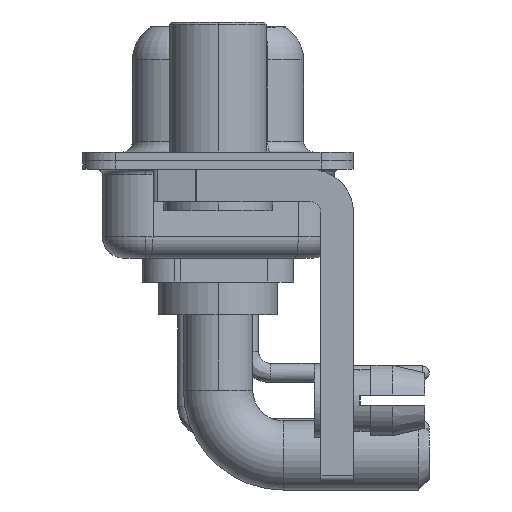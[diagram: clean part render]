
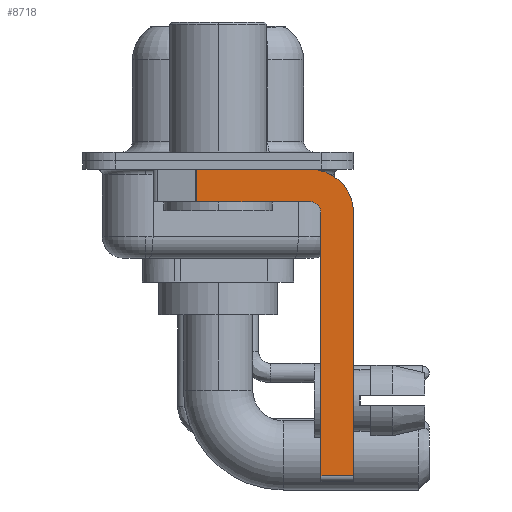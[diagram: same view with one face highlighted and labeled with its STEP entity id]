
A CAD part, left-side view. The second image highlights one B-rep face of the part: STEP entity #8718.
In plain terms, the highlighted planar face has unit normal (-1, 0, 0).
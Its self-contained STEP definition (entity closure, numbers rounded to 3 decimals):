
#2 = VECTOR ( 'NONE', #26113, 1000. ) ;
#580 = ORIENTED_EDGE ( 'NONE', *, *, #16286, .F. ) ;
#1079 = CIRCLE ( 'NONE', #10155, 2. ) ;
#2618 = DIRECTION ( 'NONE',  ( -1., 0., 0. ) ) ;
#2650 = CARTESIAN_POINT ( 'NONE',  ( -2.9, 0.978, -1.9 ) ) ;
#2651 = DIRECTION ( 'NONE',  ( 0., 0., 1. ) ) ;
#2759 = DIRECTION ( 'NONE',  ( 0., 0., -1. ) ) ;
#2904 = LINE ( 'NONE', #5308, #8463 ) ;
#2983 = ORIENTED_EDGE ( 'NONE', *, *, #18444, .F. ) ;
#3785 = DIRECTION ( 'NONE',  ( 1., 0., 0. ) ) ;
#4225 = DIRECTION ( 'NONE',  ( 0., -1., 0. ) ) ;
#4258 = VERTEX_POINT ( 'NONE', #25915 ) ;
#4605 = LINE ( 'NONE', #6196, #2 ) ;
#4687 = VERTEX_POINT ( 'NONE', #11005 ) ;
#4755 = DIRECTION ( 'NONE',  ( 0., 0., 1. ) ) ;
#4996 = CIRCLE ( 'NONE', #17217, 0.5 ) ;
#5308 = CARTESIAN_POINT ( 'NONE',  ( -2.9, 0.978, -1.9 ) ) ;
#5405 = EDGE_CURVE ( 'NONE', #19166, #7713, #22837, .T. ) ;
#5461 = EDGE_CURVE ( 'NONE', #7713, #22193, #1079, .T. ) ;
#5554 = DIRECTION ( 'NONE',  ( 0., -1., 0. ) ) ;
#6196 = CARTESIAN_POINT ( 'NONE',  ( -2.9, -6.25, -2.4 ) ) ;
#7471 = CARTESIAN_POINT ( 'NONE',  ( -2.9, -4.75, -14.8 ) ) ;
#7614 = DIRECTION ( 'NONE',  ( 0., 0., -1. ) ) ;
#7713 = VERTEX_POINT ( 'NONE', #16650 ) ;
#8463 = VECTOR ( 'NONE', #2759, 1000. ) ;
#8718 = ADVANCED_FACE ( 'NONE', ( #16398 ), #14412, .F. ) ;
#8815 = ORIENTED_EDGE ( 'NONE', *, *, #15920, .F. ) ;
#9011 = CARTESIAN_POINT ( 'NONE',  ( -2.9, -4.25, -2.4 ) ) ;
#10112 = ORIENTED_EDGE ( 'NONE', *, *, #24774, .F. ) ;
#10155 = AXIS2_PLACEMENT_3D ( 'NONE', #23113, #27479, #12633 ) ;
#10220 = CARTESIAN_POINT ( 'NONE',  ( -2.9, -6.25, -2.4 ) ) ;
#11005 = CARTESIAN_POINT ( 'NONE',  ( -2.9, -6.25, -14.55 ) ) ;
#11043 = LINE ( 'NONE', #26287, #24682 ) ;
#11050 = VECTOR ( 'NONE', #5554, 1000. ) ;
#11051 = CARTESIAN_POINT ( 'NONE',  ( -2.9, 0.978, -0.4 ) ) ;
#11721 = DIRECTION ( 'NONE',  ( 0., 1., 0. ) ) ;
#12083 = AXIS2_PLACEMENT_3D ( 'NONE', #25297, #3785, #7614 ) ;
#12367 = VERTEX_POINT ( 'NONE', #24842 ) ;
#12633 = DIRECTION ( 'NONE',  ( 0., 0., -1. ) ) ;
#13818 = VECTOR ( 'NONE', #11721, 1000. ) ;
#14412 = PLANE ( 'NONE',  #12083 ) ;
#15465 = ORIENTED_EDGE ( 'NONE', *, *, #5405, .F. ) ;
#15551 = ORIENTED_EDGE ( 'NONE', *, *, #25439, .T. ) ;
#15710 = CARTESIAN_POINT ( 'NONE',  ( -2.9, -4.25, -1.9 ) ) ;
#15920 = EDGE_CURVE ( 'NONE', #4258, #17769, #20084, .T. ) ;
#16286 = EDGE_CURVE ( 'NONE', #22193, #4687, #4605, .T. ) ;
#16398 = FACE_OUTER_BOUND ( 'NONE', #22887, .T. ) ;
#16650 = CARTESIAN_POINT ( 'NONE',  ( -2.9, -4.25, -0.4 ) ) ;
#17217 = AXIS2_PLACEMENT_3D ( 'NONE', #9011, #2618, #4755 ) ;
#17769 = VERTEX_POINT ( 'NONE', #25462 ) ;
#18152 = ORIENTED_EDGE ( 'NONE', *, *, #5461, .F. ) ;
#18444 = EDGE_CURVE ( 'NONE', #17769, #12367, #4996, .T. ) ;
#18498 = ORIENTED_EDGE ( 'NONE', *, *, #24621, .T. ) ;
#19166 = VERTEX_POINT ( 'NONE', #11051 ) ;
#20084 = LINE ( 'NONE', #7471, #23036 ) ;
#22193 = VERTEX_POINT ( 'NONE', #10220 ) ;
#22837 = LINE ( 'NONE', #24945, #11050 ) ;
#22887 = EDGE_LOOP ( 'NONE', ( #15465, #15551, #10112, #2983, #8815, #18498, #580, #18152 ) ) ;
#23036 = VECTOR ( 'NONE', #2651, 1000. ) ;
#23113 = CARTESIAN_POINT ( 'NONE',  ( -2.9, -4.25, -2.4 ) ) ;
#23449 = VERTEX_POINT ( 'NONE', #2650 ) ;
#24621 = EDGE_CURVE ( 'NONE', #4258, #4687, #11043, .T. ) ;
#24682 = VECTOR ( 'NONE', #4225, 1000. ) ;
#24774 = EDGE_CURVE ( 'NONE', #12367, #23449, #24874, .T. ) ;
#24842 = CARTESIAN_POINT ( 'NONE',  ( -2.9, -4.25, -1.9 ) ) ;
#24874 = LINE ( 'NONE', #15710, #13818 ) ;
#24945 = CARTESIAN_POINT ( 'NONE',  ( -2.9, 3., -0.4 ) ) ;
#25297 = CARTESIAN_POINT ( 'NONE',  ( -2.9, -4.25, -2.4 ) ) ;
#25439 = EDGE_CURVE ( 'NONE', #19166, #23449, #2904, .T. ) ;
#25462 = CARTESIAN_POINT ( 'NONE',  ( -2.9, -4.75, -2.4 ) ) ;
#25915 = CARTESIAN_POINT ( 'NONE',  ( -2.9, -4.75, -14.55 ) ) ;
#26113 = DIRECTION ( 'NONE',  ( 0., 0., -1. ) ) ;
#26287 = CARTESIAN_POINT ( 'NONE',  ( -2.9, -4.25, -14.55 ) ) ;
#27479 = DIRECTION ( 'NONE',  ( 1., 0., 0. ) ) ;
